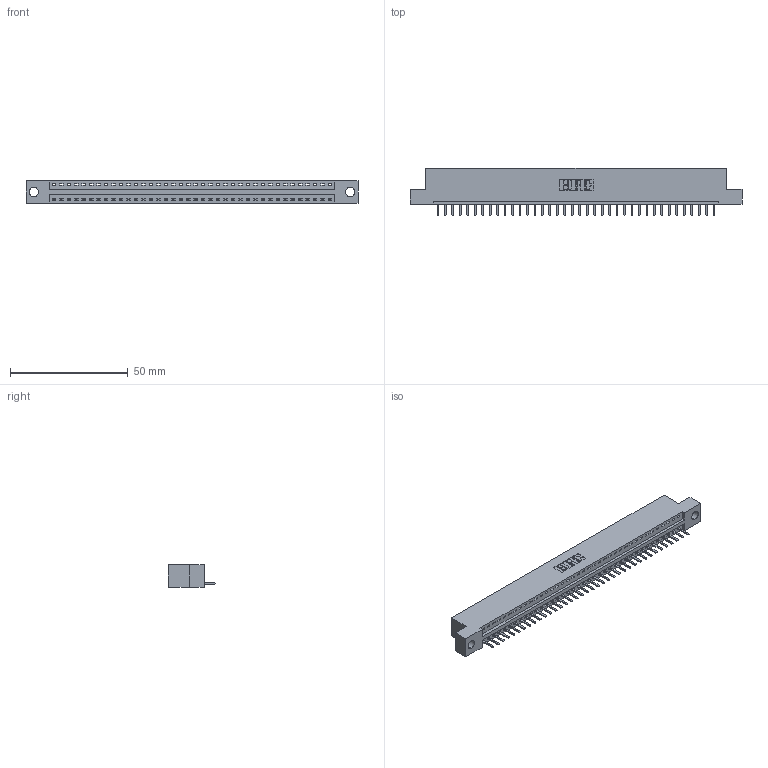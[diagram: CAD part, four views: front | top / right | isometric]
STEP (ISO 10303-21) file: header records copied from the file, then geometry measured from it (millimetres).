
FILE_DESCRIPTION (( 'STEP AP203' ), '1' );
FILE_NAME ('346-038-520-104.STEP', '2018-08-24T04:25:24', ( '' ), ( '' ), 'SwSTEP 2.0', 'SolidWorks 2016', '' );
FILE_SCHEMA (( 'CONFIG_CONTROL_DESIGN' ));
Length unit declared in the file: inch
Products named in the file (3): 346 Part_Flush Mounting Lugs - 0.156 Dia-TH; 345-292-001_345-293-120; 346-038-520-104
Assembly tree (39 placements, depth 2):
  346-038-520-104
    346 Part_Flush Mounting Lugs - 0.156 Dia-TH
    345-292-001_345-293-120  x38
Bounding box: 141.22 x 20.02 x 9.4 mm (x, y, z)
Volume: 13293.5 mm3; surface area: 16012.1 mm2
Topology: 39 solids, 39 shells, 2478 faces, 7321 edges, 4778 vertices
Faces by surface type: plane 1672, cylinder 806
Entity records: 24239 total; most frequent: CARTESIAN_POINT 4174, ORIENTED_EDGE 4134, DIRECTION 3675, EDGE_CURVE 2067, VECTOR 1779, LINE 1779, VERTEX_POINT 1374, AXIS2_PLACEMENT_3D 948
